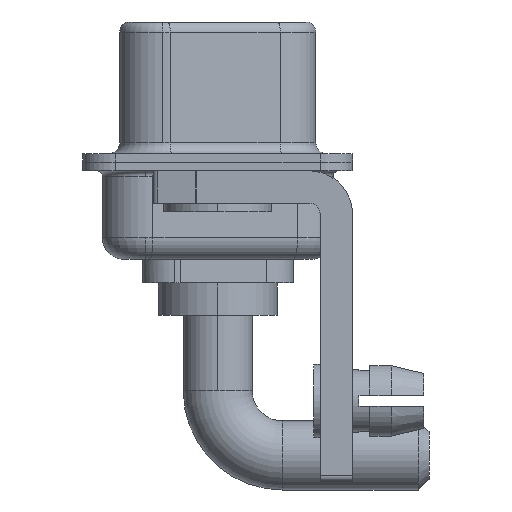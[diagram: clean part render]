
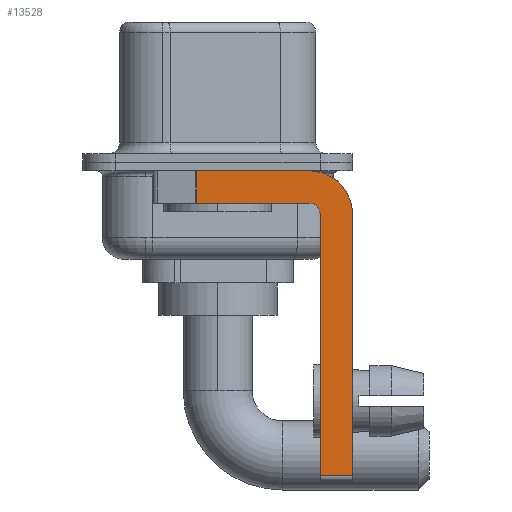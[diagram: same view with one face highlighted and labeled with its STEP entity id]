
A CAD part, left-side view. The second image highlights one B-rep face of the part: STEP entity #13528.
In plain terms, the highlighted planar face has unit normal (-1, 0, 0).
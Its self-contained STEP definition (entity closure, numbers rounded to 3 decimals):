
#163 = DIRECTION ( 'NONE',  ( 0., 0., -1. ) ) ;
#534 = EDGE_CURVE ( 'NONE', #7921, #7771, #10402, .T. ) ;
#572 = DIRECTION ( 'NONE',  ( 0., -1., 0. ) ) ;
#605 = EDGE_CURVE ( 'NONE', #3161, #4578, #14133, .T. ) ;
#655 = VECTOR ( 'NONE', #3700, 1000. ) ;
#802 = CARTESIAN_POINT ( 'NONE',  ( -2.9, -4.25, -2.4 ) ) ;
#1305 = ORIENTED_EDGE ( 'NONE', *, *, #3235, .F. ) ;
#1440 = FACE_OUTER_BOUND ( 'NONE', #5495, .T. ) ;
#2044 = DIRECTION ( 'NONE',  ( 0., 0., 1. ) ) ;
#2096 = CARTESIAN_POINT ( 'NONE',  ( -2.9, -4.25, -14.55 ) ) ;
#2405 = VECTOR ( 'NONE', #572, 1000. ) ;
#2500 = CARTESIAN_POINT ( 'NONE',  ( -2.9, 0.978, -1.9 ) ) ;
#2686 = CARTESIAN_POINT ( 'NONE',  ( -2.9, -6.25, -2.4 ) ) ;
#3001 = VERTEX_POINT ( 'NONE', #12371 ) ;
#3044 = LINE ( 'NONE', #8418, #14151 ) ;
#3161 = VERTEX_POINT ( 'NONE', #8185 ) ;
#3235 = EDGE_CURVE ( 'NONE', #12342, #4578, #4409, .T. ) ;
#3393 = EDGE_CURVE ( 'NONE', #9392, #13895, #15087, .T. ) ;
#3700 = DIRECTION ( 'NONE',  ( 0., 0., -1. ) ) ;
#3783 = DIRECTION ( 'NONE',  ( 1., 0., 0. ) ) ;
#3949 = LINE ( 'NONE', #13112, #13366 ) ;
#4409 = LINE ( 'NONE', #9304, #8587 ) ;
#4578 = VERTEX_POINT ( 'NONE', #4948 ) ;
#4948 = CARTESIAN_POINT ( 'NONE',  ( -2.9, 0.978, -1.9 ) ) ;
#5236 = LINE ( 'NONE', #2686, #7383 ) ;
#5267 = AXIS2_PLACEMENT_3D ( 'NONE', #802, #3783, #6305 ) ;
#5495 = EDGE_LOOP ( 'NONE', ( #7692, #11607, #1305, #15356, #6885, #12848, #14308, #7043 ) ) ;
#5510 = AXIS2_PLACEMENT_3D ( 'NONE', #6601, #15941, #163 ) ;
#6305 = DIRECTION ( 'NONE',  ( 0., 0., -1. ) ) ;
#6601 = CARTESIAN_POINT ( 'NONE',  ( -2.9, -4.25, -2.4 ) ) ;
#6885 = ORIENTED_EDGE ( 'NONE', *, *, #12391, .F. ) ;
#7043 = ORIENTED_EDGE ( 'NONE', *, *, #534, .F. ) ;
#7383 = VECTOR ( 'NONE', #13133, 1000. ) ;
#7692 = ORIENTED_EDGE ( 'NONE', *, *, #14636, .F. ) ;
#7771 = VERTEX_POINT ( 'NONE', #9251 ) ;
#7845 = EDGE_CURVE ( 'NONE', #3001, #12342, #11913, .T. ) ;
#7921 = VERTEX_POINT ( 'NONE', #10007 ) ;
#8015 = DIRECTION ( 'NONE',  ( 0., 1., 0. ) ) ;
#8185 = CARTESIAN_POINT ( 'NONE',  ( -2.9, 0.978, -0.4 ) ) ;
#8339 = DIRECTION ( 'NONE',  ( 0., 0., 1. ) ) ;
#8418 = CARTESIAN_POINT ( 'NONE',  ( -2.9, -4.75, -14.8 ) ) ;
#8587 = VECTOR ( 'NONE', #8015, 1000. ) ;
#9251 = CARTESIAN_POINT ( 'NONE',  ( -2.9, -6.25, -2.4 ) ) ;
#9304 = CARTESIAN_POINT ( 'NONE',  ( -2.9, -4.25, -1.9 ) ) ;
#9392 = VERTEX_POINT ( 'NONE', #13494 ) ;
#9792 = CARTESIAN_POINT ( 'NONE',  ( -2.9, -4.25, -1.9 ) ) ;
#10007 = CARTESIAN_POINT ( 'NONE',  ( -2.9, -4.25, -0.4 ) ) ;
#10402 = CIRCLE ( 'NONE', #5267, 2. ) ;
#10954 = DIRECTION ( 'NONE',  ( -1., 0., 0. ) ) ;
#11271 = CARTESIAN_POINT ( 'NONE',  ( -2.9, -4.25, -2.4 ) ) ;
#11607 = ORIENTED_EDGE ( 'NONE', *, *, #605, .T. ) ;
#11633 = AXIS2_PLACEMENT_3D ( 'NONE', #11271, #10954, #2044 ) ;
#11913 = CIRCLE ( 'NONE', #11633, 0.5 ) ;
#12039 = PLANE ( 'NONE',  #5510 ) ;
#12342 = VERTEX_POINT ( 'NONE', #9792 ) ;
#12371 = CARTESIAN_POINT ( 'NONE',  ( -2.9, -4.75, -2.4 ) ) ;
#12391 = EDGE_CURVE ( 'NONE', #9392, #3001, #3044, .T. ) ;
#12848 = ORIENTED_EDGE ( 'NONE', *, *, #3393, .T. ) ;
#13112 = CARTESIAN_POINT ( 'NONE',  ( -2.9, 3., -0.4 ) ) ;
#13133 = DIRECTION ( 'NONE',  ( 0., 0., -1. ) ) ;
#13366 = VECTOR ( 'NONE', #15483, 1000. ) ;
#13494 = CARTESIAN_POINT ( 'NONE',  ( -2.9, -4.75, -14.55 ) ) ;
#13528 = ADVANCED_FACE ( 'NONE', ( #1440 ), #12039, .F. ) ;
#13710 = CARTESIAN_POINT ( 'NONE',  ( -2.9, -6.25, -14.55 ) ) ;
#13895 = VERTEX_POINT ( 'NONE', #13710 ) ;
#14133 = LINE ( 'NONE', #2500, #655 ) ;
#14151 = VECTOR ( 'NONE', #8339, 1000. ) ;
#14308 = ORIENTED_EDGE ( 'NONE', *, *, #15469, .F. ) ;
#14636 = EDGE_CURVE ( 'NONE', #3161, #7921, #3949, .T. ) ;
#15087 = LINE ( 'NONE', #2096, #2405 ) ;
#15356 = ORIENTED_EDGE ( 'NONE', *, *, #7845, .F. ) ;
#15469 = EDGE_CURVE ( 'NONE', #7771, #13895, #5236, .T. ) ;
#15483 = DIRECTION ( 'NONE',  ( 0., -1., 0. ) ) ;
#15941 = DIRECTION ( 'NONE',  ( 1., 0., 0. ) ) ;
